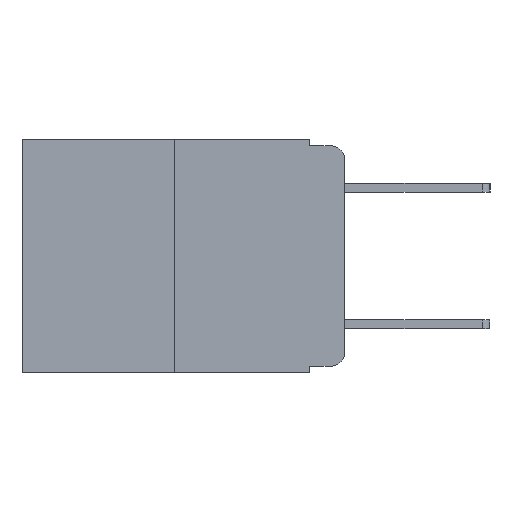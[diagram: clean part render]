
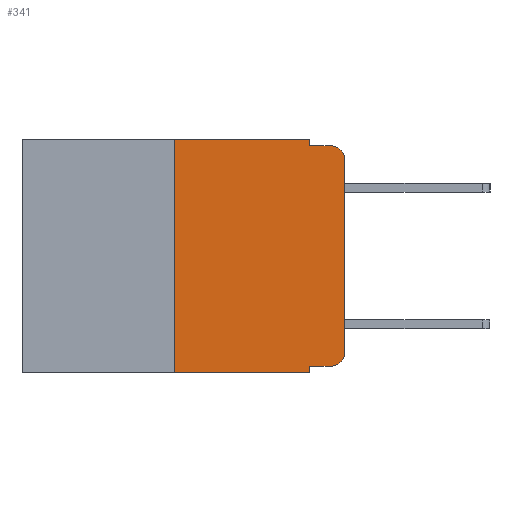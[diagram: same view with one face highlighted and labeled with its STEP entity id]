
A CAD part, left-side view. The second image highlights one B-rep face of the part: STEP entity #341.
In plain terms, the highlighted planar face has unit normal (-1, 0, 0).
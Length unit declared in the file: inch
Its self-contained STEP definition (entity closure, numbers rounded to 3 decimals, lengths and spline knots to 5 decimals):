
#38 = ORIENTED_EDGE ( 'NONE', *, *, #11003, .F. ) ;
#108 = ORIENTED_EDGE ( 'NONE', *, *, #6067, .F. ) ;
#188 = ORIENTED_EDGE ( 'NONE', *, *, #9497, .T. ) ;
#251 = AXIS2_PLACEMENT_3D ( 'NONE', #4473, #10800, #1997 ) ;
#341 = ADVANCED_FACE ( 'NONE', ( #3102 ), #1573, .F. ) ;
#663 = VECTOR ( 'NONE', #7230, 39.37008 ) ;
#727 = VECTOR ( 'NONE', #5278, 39.37008 ) ;
#766 = VECTOR ( 'NONE', #7229, 39.37008 ) ;
#935 = DIRECTION ( 'NONE',  ( 0., -1., 0. ) ) ;
#1137 = DIRECTION ( 'NONE',  ( 1., 0., 0. ) ) ;
#1189 = CIRCLE ( 'NONE', #251, 0.02 ) ;
#1237 = DIRECTION ( 'NONE',  ( 0., 0., -1. ) ) ;
#1452 = VERTEX_POINT ( 'NONE', #2994 ) ;
#1470 = VERTEX_POINT ( 'NONE', #5410 ) ;
#1527 = ORIENTED_EDGE ( 'NONE', *, *, #8684, .F. ) ;
#1573 = PLANE ( 'NONE',  #9146 ) ;
#1856 = CARTESIAN_POINT ( 'NONE',  ( 0., 0., -0.03 ) ) ;
#1898 = CARTESIAN_POINT ( 'NONE',  ( 0., 0.051, -0.01 ) ) ;
#1997 = DIRECTION ( 'NONE',  ( 0., 0., -1. ) ) ;
#2035 = EDGE_CURVE ( 'NONE', #2434, #1452, #9334, .T. ) ;
#2284 = VERTEX_POINT ( 'NONE', #10291 ) ;
#2434 = VERTEX_POINT ( 'NONE', #11120 ) ;
#2694 = CARTESIAN_POINT ( 'NONE',  ( 0., 0.473, -0.343 ) ) ;
#2756 = VECTOR ( 'NONE', #6570, 39.37008 ) ;
#2933 = ORIENTED_EDGE ( 'NONE', *, *, #3371, .T. ) ;
#2994 = CARTESIAN_POINT ( 'NONE',  ( 0., 0.25, 0. ) ) ;
#3102 = FACE_OUTER_BOUND ( 'NONE', #6596, .T. ) ;
#3265 = LINE ( 'NONE', #6377, #663 ) ;
#3371 = EDGE_CURVE ( 'NONE', #4051, #9265, #1189, .T. ) ;
#3500 = CARTESIAN_POINT ( 'NONE',  ( 0., 0.051, -0.343 ) ) ;
#3676 = CARTESIAN_POINT ( 'NONE',  ( 0., 0.02, -0.01 ) ) ;
#3821 = ORIENTED_EDGE ( 'NONE', *, *, #2035, .F. ) ;
#4051 = VERTEX_POINT ( 'NONE', #1856 ) ;
#4083 = VECTOR ( 'NONE', #5421, 39.37008 ) ;
#4459 = ORIENTED_EDGE ( 'NONE', *, *, #5882, .T. ) ;
#4473 = CARTESIAN_POINT ( 'NONE',  ( 0., 0.02, -0.03 ) ) ;
#4594 = CARTESIAN_POINT ( 'NONE',  ( 0., 0.051, -0.333 ) ) ;
#4773 = ORIENTED_EDGE ( 'NONE', *, *, #10038, .T. ) ;
#4810 = LINE ( 'NONE', #2694, #11327 ) ;
#4865 = CARTESIAN_POINT ( 'NONE',  ( 0., 0.02, -0.313 ) ) ;
#5227 = VECTOR ( 'NONE', #8369, 39.37008 ) ;
#5278 = DIRECTION ( 'NONE',  ( 0., 0., -1. ) ) ;
#5410 = CARTESIAN_POINT ( 'NONE',  ( 0., 0.02, -0.333 ) ) ;
#5421 = DIRECTION ( 'NONE',  ( 0., 0., 1. ) ) ;
#5501 = CARTESIAN_POINT ( 'NONE',  ( 0., 0.25, 0. ) ) ;
#5679 = CARTESIAN_POINT ( 'NONE',  ( 0., 0.051, 0. ) ) ;
#5726 = LINE ( 'NONE', #7267, #766 ) ;
#5748 = DIRECTION ( 'NONE',  ( 0., 0., -1. ) ) ;
#5882 = EDGE_CURVE ( 'NONE', #2434, #7329, #4810, .T. ) ;
#6067 = EDGE_CURVE ( 'NONE', #1452, #7651, #7243, .T. ) ;
#6073 = ORIENTED_EDGE ( 'NONE', *, *, #6527, .T. ) ;
#6377 = CARTESIAN_POINT ( 'NONE',  ( 0., 0.051, -0.333 ) ) ;
#6487 = ORIENTED_EDGE ( 'NONE', *, *, #8801, .F. ) ;
#6527 = EDGE_CURVE ( 'NONE', #7444, #1470, #3265, .T. ) ;
#6570 = DIRECTION ( 'NONE',  ( 0., 0., -1. ) ) ;
#6596 = EDGE_LOOP ( 'NONE', ( #4773, #2933, #1527, #6487, #108, #3821, #4459, #38, #6073, #188 ) ) ;
#6666 = CARTESIAN_POINT ( 'NONE',  ( 0., 0.051, 0. ) ) ;
#7229 = DIRECTION ( 'NONE',  ( 0., -1., 0. ) ) ;
#7230 = DIRECTION ( 'NONE',  ( 0., -1., 0. ) ) ;
#7243 = LINE ( 'NONE', #10017, #5227 ) ;
#7267 = CARTESIAN_POINT ( 'NONE',  ( 0., 0.051, -0.01 ) ) ;
#7329 = VERTEX_POINT ( 'NONE', #3500 ) ;
#7350 = VECTOR ( 'NONE', #8312, 39.37008 ) ;
#7370 = AXIS2_PLACEMENT_3D ( 'NONE', #4865, #10815, #5748 ) ;
#7444 = VERTEX_POINT ( 'NONE', #4594 ) ;
#7651 = VERTEX_POINT ( 'NONE', #6666 ) ;
#7719 = LINE ( 'NONE', #11204, #727 ) ;
#8201 = VERTEX_POINT ( 'NONE', #1898 ) ;
#8312 = DIRECTION ( 'NONE',  ( 0., 0., 1. ) ) ;
#8369 = DIRECTION ( 'NONE',  ( 0., -1., 0. ) ) ;
#8413 = LINE ( 'NONE', #9684, #4083 ) ;
#8684 = EDGE_CURVE ( 'NONE', #8201, #9265, #5726, .T. ) ;
#8801 = EDGE_CURVE ( 'NONE', #7651, #8201, #11408, .T. ) ;
#9146 = AXIS2_PLACEMENT_3D ( 'NONE', #9239, #1137, #1237 ) ;
#9239 = CARTESIAN_POINT ( 'NONE',  ( 0., 0.473, 0. ) ) ;
#9265 = VERTEX_POINT ( 'NONE', #3676 ) ;
#9334 = LINE ( 'NONE', #5501, #7350 ) ;
#9497 = EDGE_CURVE ( 'NONE', #1470, #2284, #9970, .T. ) ;
#9684 = CARTESIAN_POINT ( 'NONE',  ( 0., 0., 0. ) ) ;
#9970 = CIRCLE ( 'NONE', #7370, 0.02 ) ;
#10017 = CARTESIAN_POINT ( 'NONE',  ( 0., 0.473, 0. ) ) ;
#10038 = EDGE_CURVE ( 'NONE', #2284, #4051, #8413, .T. ) ;
#10291 = CARTESIAN_POINT ( 'NONE',  ( 0., 0., -0.313 ) ) ;
#10800 = DIRECTION ( 'NONE',  ( -1., 0., 0. ) ) ;
#10815 = DIRECTION ( 'NONE',  ( -1., 0., 0. ) ) ;
#11003 = EDGE_CURVE ( 'NONE', #7444, #7329, #7719, .T. ) ;
#11120 = CARTESIAN_POINT ( 'NONE',  ( 0., 0.25, -0.343 ) ) ;
#11204 = CARTESIAN_POINT ( 'NONE',  ( 0., 0.051, 0. ) ) ;
#11327 = VECTOR ( 'NONE', #935, 39.37008 ) ;
#11408 = LINE ( 'NONE', #5679, #2756 ) ;
